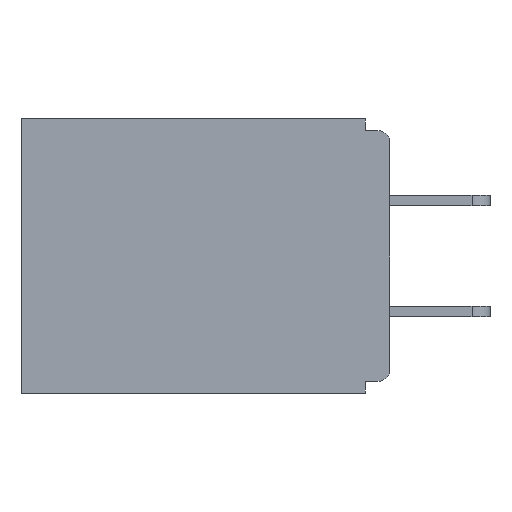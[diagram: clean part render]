
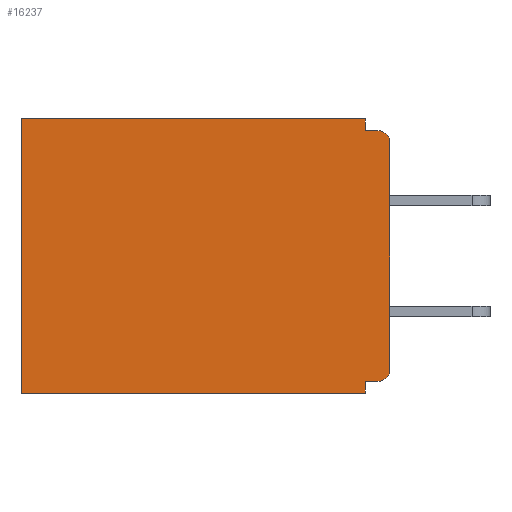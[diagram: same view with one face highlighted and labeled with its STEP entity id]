
A CAD part, left-side view. The second image highlights one B-rep face of the part: STEP entity #16237.
In plain terms, the highlighted planar face has unit normal (-1, 0, 0).
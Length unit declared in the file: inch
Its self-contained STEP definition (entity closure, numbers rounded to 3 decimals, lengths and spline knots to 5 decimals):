
#475 = ORIENTED_EDGE ( 'NONE', *, *, #12655, .T. ) ;
#1057 = VERTEX_POINT ( 'NONE', #13535 ) ;
#2579 = PLANE ( 'NONE',  #7734 ) ;
#3039 = VECTOR ( 'NONE', #8387, 39.37008 ) ;
#3527 = VECTOR ( 'NONE', #18997, 39.37008 ) ;
#3615 = EDGE_CURVE ( 'NONE', #12887, #8593, #6134, .T. ) ;
#4387 = LINE ( 'NONE', #23495, #22864 ) ;
#4388 = CARTESIAN_POINT ( 'NONE',  ( 0.298, 0., 0. ) ) ;
#4613 = CARTESIAN_POINT ( 'NONE',  ( 0.298, 0.031, -0.343 ) ) ;
#4914 = CARTESIAN_POINT ( 'NONE',  ( 0.298, 0., 0. ) ) ;
#5236 = DIRECTION ( 'NONE',  ( 0., 1., 0. ) ) ;
#5655 = VERTEX_POINT ( 'NONE', #4613 ) ;
#5754 = AXIS2_PLACEMENT_3D ( 'NONE', #18950, #24642, #8708 ) ;
#5825 = FACE_OUTER_BOUND ( 'NONE', #23574, .T. ) ;
#6134 = LINE ( 'NONE', #9289, #12065 ) ;
#6348 = LINE ( 'NONE', #4914, #22016 ) ;
#6554 = CARTESIAN_POINT ( 'NONE',  ( 0.298, 0.46, 0. ) ) ;
#6702 = VERTEX_POINT ( 'NONE', #6554 ) ;
#6960 = EDGE_CURVE ( 'NONE', #22188, #1057, #20072, .T. ) ;
#7214 = CARTESIAN_POINT ( 'NONE',  ( 0.298, 0.015, -0.015 ) ) ;
#7424 = CARTESIAN_POINT ( 'NONE',  ( 0.298, 0.031, -0.328 ) ) ;
#7734 = AXIS2_PLACEMENT_3D ( 'NONE', #16519, #22266, #20565 ) ;
#7855 = VERTEX_POINT ( 'NONE', #24070 ) ;
#7944 = CIRCLE ( 'NONE', #5754, 0.015 ) ;
#8229 = ORIENTED_EDGE ( 'NONE', *, *, #17938, .F. ) ;
#8387 = DIRECTION ( 'NONE',  ( 0., 0., -1. ) ) ;
#8593 = VERTEX_POINT ( 'NONE', #7424 ) ;
#8708 = DIRECTION ( 'NONE',  ( 0., 0., -1. ) ) ;
#8945 = DIRECTION ( 'NONE',  ( 0., 0., -1. ) ) ;
#8951 = LINE ( 'NONE', #4388, #3039 ) ;
#8971 = EDGE_CURVE ( 'NONE', #6702, #16457, #24958, .T. ) ;
#9118 = CARTESIAN_POINT ( 'NONE',  ( 0.298, 0.015, -0.313 ) ) ;
#9130 = EDGE_CURVE ( 'NONE', #12887, #7855, #12129, .T. ) ;
#9289 = CARTESIAN_POINT ( 'NONE',  ( 0.298, 0., -0.328 ) ) ;
#9445 = LINE ( 'NONE', #14907, #11335 ) ;
#9593 = DIRECTION ( 'NONE',  ( 0., 0., -1. ) ) ;
#10634 = ORIENTED_EDGE ( 'NONE', *, *, #23244, .F. ) ;
#11335 = VECTOR ( 'NONE', #5236, 39.37008 ) ;
#12065 = VECTOR ( 'NONE', #17785, 39.37008 ) ;
#12129 = CIRCLE ( 'NONE', #17993, 0.015 ) ;
#12655 = EDGE_CURVE ( 'NONE', #22188, #6702, #6348, .T. ) ;
#12757 = DIRECTION ( 'NONE',  ( 0., 1., 0. ) ) ;
#12887 = VERTEX_POINT ( 'NONE', #18482 ) ;
#13150 = EDGE_CURVE ( 'NONE', #8593, #5655, #19151, .T. ) ;
#13339 = VERTEX_POINT ( 'NONE', #24580 ) ;
#13535 = CARTESIAN_POINT ( 'NONE',  ( 0.298, 0.031, -0.015 ) ) ;
#14230 = ORIENTED_EDGE ( 'NONE', *, *, #8971, .T. ) ;
#14907 = CARTESIAN_POINT ( 'NONE',  ( 0.298, 0., -0.343 ) ) ;
#15154 = CARTESIAN_POINT ( 'NONE',  ( 0.298, 0.46, 0. ) ) ;
#15196 = CARTESIAN_POINT ( 'NONE',  ( 0.298, 0.031, -0.343 ) ) ;
#15542 = ORIENTED_EDGE ( 'NONE', *, *, #6960, .F. ) ;
#16237 = ADVANCED_FACE ( 'NONE', ( #5825 ), #2579, .F. ) ;
#16457 = VERTEX_POINT ( 'NONE', #24132 ) ;
#16519 = CARTESIAN_POINT ( 'NONE',  ( 0.298, 0., 0. ) ) ;
#16895 = DIRECTION ( 'NONE',  ( -1., 0., 0. ) ) ;
#17142 = EDGE_CURVE ( 'NONE', #13339, #20082, #7944, .T. ) ;
#17785 = DIRECTION ( 'NONE',  ( 0., 1., 0. ) ) ;
#17938 = EDGE_CURVE ( 'NONE', #5655, #16457, #9445, .T. ) ;
#17993 = AXIS2_PLACEMENT_3D ( 'NONE', #9118, #16895, #8945 ) ;
#18482 = CARTESIAN_POINT ( 'NONE',  ( 0.298, 0.015, -0.328 ) ) ;
#18716 = VECTOR ( 'NONE', #9593, 39.37008 ) ;
#18761 = ORIENTED_EDGE ( 'NONE', *, *, #3615, .F. ) ;
#18950 = CARTESIAN_POINT ( 'NONE',  ( 0.298, 0.015, -0.03 ) ) ;
#18997 = DIRECTION ( 'NONE',  ( 0., 0., -1. ) ) ;
#19128 = VECTOR ( 'NONE', #25605, 39.37008 ) ;
#19151 = LINE ( 'NONE', #15196, #3527 ) ;
#19483 = CARTESIAN_POINT ( 'NONE',  ( 0.298, 0.031, -0.343 ) ) ;
#20072 = LINE ( 'NONE', #19483, #19128 ) ;
#20082 = VERTEX_POINT ( 'NONE', #7214 ) ;
#20565 = DIRECTION ( 'NONE',  ( 0., 0., -1. ) ) ;
#20893 = ORIENTED_EDGE ( 'NONE', *, *, #9130, .T. ) ;
#22016 = VECTOR ( 'NONE', #12757, 39.37008 ) ;
#22188 = VERTEX_POINT ( 'NONE', #23459 ) ;
#22266 = DIRECTION ( 'NONE',  ( 1., 0., 0. ) ) ;
#22500 = ORIENTED_EDGE ( 'NONE', *, *, #25387, .F. ) ;
#22864 = VECTOR ( 'NONE', #23676, 39.37008 ) ;
#23045 = ORIENTED_EDGE ( 'NONE', *, *, #17142, .T. ) ;
#23244 = EDGE_CURVE ( 'NONE', #1057, #20082, #4387, .T. ) ;
#23459 = CARTESIAN_POINT ( 'NONE',  ( 0.298, 0.031, 0. ) ) ;
#23495 = CARTESIAN_POINT ( 'NONE',  ( 0.298, 0., -0.015 ) ) ;
#23574 = EDGE_LOOP ( 'NONE', ( #23045, #10634, #15542, #475, #14230, #8229, #25762, #18761, #20893, #22500 ) ) ;
#23676 = DIRECTION ( 'NONE',  ( 0., -1., 0. ) ) ;
#24070 = CARTESIAN_POINT ( 'NONE',  ( 0.298, 0., -0.313 ) ) ;
#24132 = CARTESIAN_POINT ( 'NONE',  ( 0.298, 0.46, -0.343 ) ) ;
#24580 = CARTESIAN_POINT ( 'NONE',  ( 0.298, 0., -0.03 ) ) ;
#24642 = DIRECTION ( 'NONE',  ( -1., 0., 0. ) ) ;
#24958 = LINE ( 'NONE', #15154, #18716 ) ;
#25387 = EDGE_CURVE ( 'NONE', #13339, #7855, #8951, .T. ) ;
#25605 = DIRECTION ( 'NONE',  ( 0., 0., -1. ) ) ;
#25762 = ORIENTED_EDGE ( 'NONE', *, *, #13150, .F. ) ;
